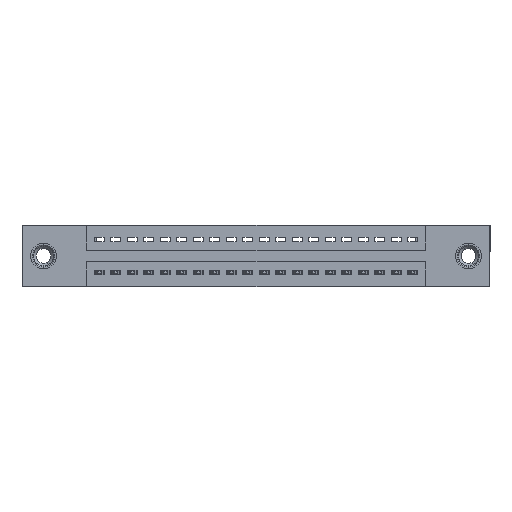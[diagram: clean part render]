
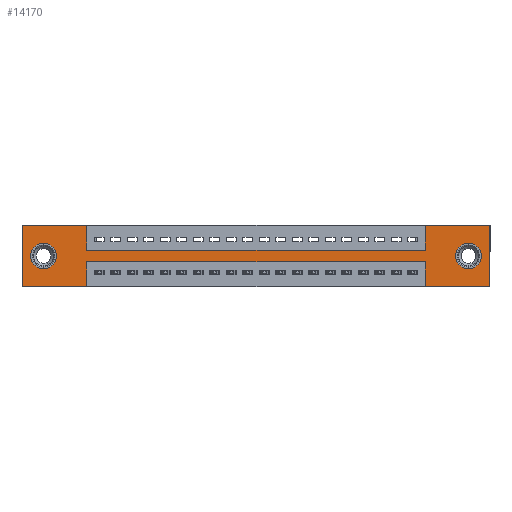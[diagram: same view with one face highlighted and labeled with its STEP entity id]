
A CAD part, front view. The second image highlights one B-rep face of the part: STEP entity #14170.
In plain terms, the highlighted planar face has unit normal (0, -1, 0).
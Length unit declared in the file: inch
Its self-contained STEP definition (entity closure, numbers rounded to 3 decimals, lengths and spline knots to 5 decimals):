
#97 = LINE ( 'NONE', #17802, #10287 ) ;
#153 = ORIENTED_EDGE ( 'NONE', *, *, #13393, .T. ) ;
#158 = VERTEX_POINT ( 'NONE', #5447 ) ;
#263 = VECTOR ( 'NONE', #10149, 39.37008 ) ;
#452 = AXIS2_PLACEMENT_3D ( 'NONE', #20174, #12098, #13843 ) ;
#468 = ORIENTED_EDGE ( 'NONE', *, *, #12521, .F. ) ;
#823 = AXIS2_PLACEMENT_3D ( 'NONE', #7329, #1293, #16897 ) ;
#875 = VECTOR ( 'NONE', #19132, 39.37008 ) ;
#1293 = DIRECTION ( 'NONE',  ( 0., 1., 0. ) ) ;
#1296 = CARTESIAN_POINT ( 'NONE',  ( 0.13, 0., -0.107 ) ) ;
#1312 = ORIENTED_EDGE ( 'NONE', *, *, #4836, .T. ) ;
#1349 = DIRECTION ( 'NONE',  ( -1., 0., 0. ) ) ;
#1374 = CARTESIAN_POINT ( 'NONE',  ( 0., 0., -0.37 ) ) ;
#1524 = EDGE_CURVE ( 'NONE', #16544, #2745, #16502, .T. ) ;
#1643 = FACE_OUTER_BOUND ( 'NONE', #17632, .T. ) ;
#1860 = VERTEX_POINT ( 'NONE', #6330 ) ;
#1952 = ORIENTED_EDGE ( 'NONE', *, *, #4132, .F. ) ;
#2158 = DIRECTION ( 'NONE',  ( 0., 0., -1. ) ) ;
#2629 = LINE ( 'NONE', #17013, #6470 ) ;
#2745 = VERTEX_POINT ( 'NONE', #3622 ) ;
#2796 = CARTESIAN_POINT ( 'NONE',  ( 2.705, 0., -0.185 ) ) ;
#2922 = CARTESIAN_POINT ( 'NONE',  ( 0.3925, 0., -0.22 ) ) ;
#3301 = CIRCLE ( 'NONE', #11587, 0.078 ) ;
#3545 = CARTESIAN_POINT ( 'NONE',  ( 0.3925, 0., -0.37 ) ) ;
#3622 = CARTESIAN_POINT ( 'NONE',  ( 2.4425, 0., -0.37 ) ) ;
#3797 = VERTEX_POINT ( 'NONE', #5092 ) ;
#3877 = EDGE_CURVE ( 'NONE', #16101, #17182, #15176, .T. ) ;
#4132 = EDGE_CURVE ( 'NONE', #12563, #12225, #5864, .T. ) ;
#4174 = CARTESIAN_POINT ( 'NONE',  ( 2.705, 0., -0.263 ) ) ;
#4224 = ORIENTED_EDGE ( 'NONE', *, *, #3877, .T. ) ;
#4231 = CARTESIAN_POINT ( 'NONE',  ( 2.705, 0., -0.107 ) ) ;
#4344 = LINE ( 'NONE', #10304, #13098 ) ;
#4614 = LINE ( 'NONE', #18343, #16085 ) ;
#4836 = EDGE_CURVE ( 'NONE', #158, #10678, #16833, .T. ) ;
#4915 = ORIENTED_EDGE ( 'NONE', *, *, #5492, .F. ) ;
#5092 = CARTESIAN_POINT ( 'NONE',  ( 0., 0., 0. ) ) ;
#5447 = CARTESIAN_POINT ( 'NONE',  ( 0.13, 0., -0.263 ) ) ;
#5487 = LINE ( 'NONE', #16225, #875 ) ;
#5492 = EDGE_CURVE ( 'NONE', #11634, #9446, #13384, .T. ) ;
#5493 = ORIENTED_EDGE ( 'NONE', *, *, #1524, .F. ) ;
#5505 = VECTOR ( 'NONE', #14416, 39.37008 ) ;
#5664 = ORIENTED_EDGE ( 'NONE', *, *, #12013, .F. ) ;
#5765 = FACE_BOUND ( 'NONE', #9383, .T. ) ;
#5864 = LINE ( 'NONE', #10970, #13703 ) ;
#6038 = VECTOR ( 'NONE', #8696, 39.37008 ) ;
#6067 = CARTESIAN_POINT ( 'NONE',  ( 0.3925, 0., -0.37 ) ) ;
#6079 = DIRECTION ( 'NONE',  ( 0., 1., 0. ) ) ;
#6330 = CARTESIAN_POINT ( 'NONE',  ( 2.4425, 0., 0. ) ) ;
#6355 = ORIENTED_EDGE ( 'NONE', *, *, #7898, .T. ) ;
#6403 = ORIENTED_EDGE ( 'NONE', *, *, #11707, .F. ) ;
#6453 = ORIENTED_EDGE ( 'NONE', *, *, #9967, .F. ) ;
#6470 = VECTOR ( 'NONE', #12432, 39.37008 ) ;
#6703 = VECTOR ( 'NONE', #10790, 39.37008 ) ;
#7102 = VERTEX_POINT ( 'NONE', #15875 ) ;
#7329 = CARTESIAN_POINT ( 'NONE',  ( 0.13, 0., -0.185 ) ) ;
#7898 = EDGE_CURVE ( 'NONE', #10678, #158, #12499, .T. ) ;
#8442 = CARTESIAN_POINT ( 'NONE',  ( 0., 0., -0.37 ) ) ;
#8542 = DIRECTION ( 'NONE',  ( 0., 0., 1. ) ) ;
#8580 = CARTESIAN_POINT ( 'NONE',  ( 0., 0., 0. ) ) ;
#8696 = DIRECTION ( 'NONE',  ( 1., 0., 0. ) ) ;
#9274 = CARTESIAN_POINT ( 'NONE',  ( 0., 0., -0.37 ) ) ;
#9383 = EDGE_LOOP ( 'NONE', ( #153, #4224 ) ) ;
#9385 = VERTEX_POINT ( 'NONE', #14800 ) ;
#9446 = VERTEX_POINT ( 'NONE', #11955 ) ;
#9791 = PLANE ( 'NONE',  #14057 ) ;
#9967 = EDGE_CURVE ( 'NONE', #1860, #7102, #18065, .T. ) ;
#10149 = DIRECTION ( 'NONE',  ( 0., 0., 1. ) ) ;
#10189 = ORIENTED_EDGE ( 'NONE', *, *, #17161, .F. ) ;
#10287 = VECTOR ( 'NONE', #8542, 39.37008 ) ;
#10304 = CARTESIAN_POINT ( 'NONE',  ( 0., 0., 0. ) ) ;
#10512 = DIRECTION ( 'NONE',  ( 0., 0., -1. ) ) ;
#10678 = VERTEX_POINT ( 'NONE', #1296 ) ;
#10681 = ORIENTED_EDGE ( 'NONE', *, *, #19158, .F. ) ;
#10790 = DIRECTION ( 'NONE',  ( -1., 0., 0. ) ) ;
#10970 = CARTESIAN_POINT ( 'NONE',  ( 0.3925, 0., 0. ) ) ;
#11181 = VECTOR ( 'NONE', #14476, 39.37008 ) ;
#11513 = CARTESIAN_POINT ( 'NONE',  ( 0., 0., 0. ) ) ;
#11587 = AXIS2_PLACEMENT_3D ( 'NONE', #13540, #13609, #19768 ) ;
#11634 = VERTEX_POINT ( 'NONE', #6067 ) ;
#11648 = EDGE_CURVE ( 'NONE', #12225, #11684, #2629, .T. ) ;
#11684 = VERTEX_POINT ( 'NONE', #16511 ) ;
#11707 = EDGE_CURVE ( 'NONE', #9446, #3797, #4344, .T. ) ;
#11955 = CARTESIAN_POINT ( 'NONE',  ( 0., 0., -0.37 ) ) ;
#12013 = EDGE_CURVE ( 'NONE', #12930, #11634, #19184, .T. ) ;
#12098 = DIRECTION ( 'NONE',  ( 0., 1., 0. ) ) ;
#12225 = VERTEX_POINT ( 'NONE', #18516 ) ;
#12432 = DIRECTION ( 'NONE',  ( 1., 0., 0. ) ) ;
#12499 = CIRCLE ( 'NONE', #452, 0.078 ) ;
#12521 = EDGE_CURVE ( 'NONE', #9385, #12930, #5487, .T. ) ;
#12563 = VERTEX_POINT ( 'NONE', #16475 ) ;
#12572 = DIRECTION ( 'NONE',  ( 0., 0., -1. ) ) ;
#12696 = LINE ( 'NONE', #19772, #263 ) ;
#12930 = VERTEX_POINT ( 'NONE', #2922 ) ;
#12968 = DIRECTION ( 'NONE',  ( 0., -1., 0. ) ) ;
#13098 = VECTOR ( 'NONE', #13565, 39.37008 ) ;
#13384 = LINE ( 'NONE', #9274, #15345 ) ;
#13393 = EDGE_CURVE ( 'NONE', #17182, #16101, #3301, .T. ) ;
#13540 = CARTESIAN_POINT ( 'NONE',  ( 2.705, 0., -0.185 ) ) ;
#13565 = DIRECTION ( 'NONE',  ( 0., 0., 1. ) ) ;
#13609 = DIRECTION ( 'NONE',  ( 0., 1., 0. ) ) ;
#13703 = VECTOR ( 'NONE', #12572, 39.37008 ) ;
#13843 = DIRECTION ( 'NONE',  ( 0., 0., 1. ) ) ;
#13891 = DIRECTION ( 'NONE',  ( 0., 0., -1. ) ) ;
#14057 = AXIS2_PLACEMENT_3D ( 'NONE', #8442, #12968, #2158 ) ;
#14170 = ADVANCED_FACE ( 'NONE', ( #5765, #19450, #1643 ), #9791, .T. ) ;
#14346 = LINE ( 'NONE', #8580, #6038 ) ;
#14416 = DIRECTION ( 'NONE',  ( 0., 0., -1. ) ) ;
#14476 = DIRECTION ( 'NONE',  ( 1., 0., 0. ) ) ;
#14800 = CARTESIAN_POINT ( 'NONE',  ( 2.4425, 0., -0.22 ) ) ;
#14922 = AXIS2_PLACEMENT_3D ( 'NONE', #2796, #6079, #13891 ) ;
#14959 = ORIENTED_EDGE ( 'NONE', *, *, #19870, .F. ) ;
#15176 = CIRCLE ( 'NONE', #14922, 0.078 ) ;
#15345 = VECTOR ( 'NONE', #1349, 39.37008 ) ;
#15875 = CARTESIAN_POINT ( 'NONE',  ( 2.835, 0., 0. ) ) ;
#15947 = CARTESIAN_POINT ( 'NONE',  ( 2.835, 0., -0.37 ) ) ;
#15996 = EDGE_CURVE ( 'NONE', #11684, #1860, #97, .T. ) ;
#16085 = VECTOR ( 'NONE', #10512, 39.37008 ) ;
#16101 = VERTEX_POINT ( 'NONE', #4174 ) ;
#16225 = CARTESIAN_POINT ( 'NONE',  ( 0.3925, 0., -0.22 ) ) ;
#16249 = EDGE_LOOP ( 'NONE', ( #6355, #1312 ) ) ;
#16475 = CARTESIAN_POINT ( 'NONE',  ( 0.3925, 0., 0. ) ) ;
#16502 = LINE ( 'NONE', #1374, #6703 ) ;
#16511 = CARTESIAN_POINT ( 'NONE',  ( 2.4425, 0., -0.15 ) ) ;
#16544 = VERTEX_POINT ( 'NONE', #15947 ) ;
#16833 = CIRCLE ( 'NONE', #823, 0.078 ) ;
#16897 = DIRECTION ( 'NONE',  ( 0., 0., 1. ) ) ;
#16979 = ORIENTED_EDGE ( 'NONE', *, *, #11648, .F. ) ;
#17013 = CARTESIAN_POINT ( 'NONE',  ( 0.3925, 0., -0.15 ) ) ;
#17161 = EDGE_CURVE ( 'NONE', #2745, #9385, #12696, .T. ) ;
#17182 = VERTEX_POINT ( 'NONE', #4231 ) ;
#17632 = EDGE_LOOP ( 'NONE', ( #5664, #468, #10189, #5493, #14959, #6453, #18366, #16979, #1952, #10681, #6403, #4915 ) ) ;
#17802 = CARTESIAN_POINT ( 'NONE',  ( 2.4425, 0., 0. ) ) ;
#18065 = LINE ( 'NONE', #11513, #11181 ) ;
#18343 = CARTESIAN_POINT ( 'NONE',  ( 2.835, 0., 0. ) ) ;
#18366 = ORIENTED_EDGE ( 'NONE', *, *, #15996, .F. ) ;
#18516 = CARTESIAN_POINT ( 'NONE',  ( 0.3925, 0., -0.15 ) ) ;
#19132 = DIRECTION ( 'NONE',  ( -1., 0., 0. ) ) ;
#19158 = EDGE_CURVE ( 'NONE', #3797, #12563, #14346, .T. ) ;
#19184 = LINE ( 'NONE', #3545, #5505 ) ;
#19450 = FACE_BOUND ( 'NONE', #16249, .T. ) ;
#19768 = DIRECTION ( 'NONE',  ( 0., 0., -1. ) ) ;
#19772 = CARTESIAN_POINT ( 'NONE',  ( 2.4425, 0., -0.37 ) ) ;
#19870 = EDGE_CURVE ( 'NONE', #7102, #16544, #4614, .T. ) ;
#20174 = CARTESIAN_POINT ( 'NONE',  ( 0.13, 0., -0.185 ) ) ;
